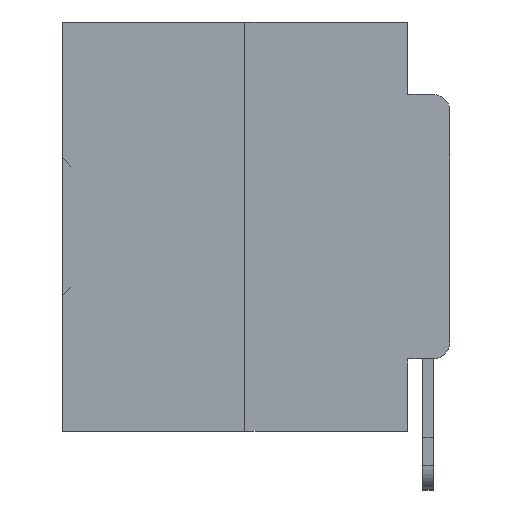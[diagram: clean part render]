
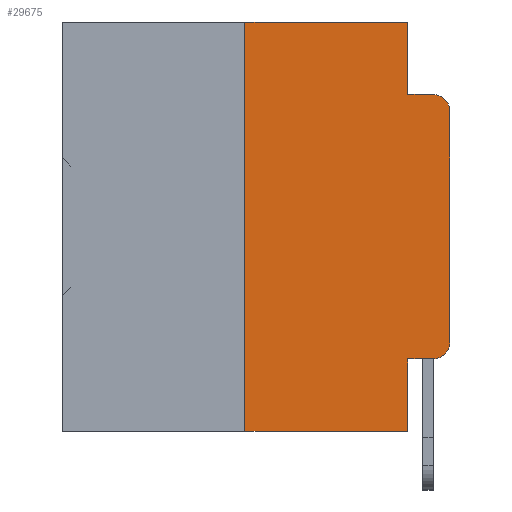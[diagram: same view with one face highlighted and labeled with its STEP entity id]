
A CAD part, left-side view. The second image highlights one B-rep face of the part: STEP entity #29675.
In plain terms, the highlighted planar face has unit normal (-1, 0, 0).
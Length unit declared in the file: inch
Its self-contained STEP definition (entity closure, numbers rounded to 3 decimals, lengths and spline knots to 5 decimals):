
#100 = DIRECTION ( 'NONE',  ( 0., 0., -1. ) ) ;
#539 = CIRCLE ( 'NONE', #15684, 0.02 ) ;
#1076 = CARTESIAN_POINT ( 'NONE',  ( 0., 0.051, 0. ) ) ;
#1246 = EDGE_CURVE ( 'NONE', #37813, #13424, #34353, .T. ) ;
#1493 = DIRECTION ( 'NONE',  ( 0., -1., 0. ) ) ;
#1650 = CARTESIAN_POINT ( 'NONE',  ( 0., 0.02, -0.0885 ) ) ;
#1823 = VERTEX_POINT ( 'NONE', #19265 ) ;
#1852 = ORIENTED_EDGE ( 'NONE', *, *, #6979, .F. ) ;
#2074 = CARTESIAN_POINT ( 'NONE',  ( 0., 0.25, -0.5 ) ) ;
#2303 = DIRECTION ( 'NONE',  ( 0., -1., 0. ) ) ;
#2508 = LINE ( 'NONE', #35994, #16537 ) ;
#2762 = ORIENTED_EDGE ( 'NONE', *, *, #8269, .T. ) ;
#3209 = DIRECTION ( 'NONE',  ( 0., 0., -1. ) ) ;
#4046 = DIRECTION ( 'NONE',  ( 0., 0., -1. ) ) ;
#4288 = ORIENTED_EDGE ( 'NONE', *, *, #35094, .T. ) ;
#4945 = EDGE_LOOP ( 'NONE', ( #7257, #2762, #1852, #21828, #7993, #10162, #32004, #15299, #10810, #4288 ) ) ;
#6101 = CARTESIAN_POINT ( 'NONE',  ( 0., 0.473, 0. ) ) ;
#6979 = EDGE_CURVE ( 'NONE', #8449, #25512, #19978, .T. ) ;
#7257 = ORIENTED_EDGE ( 'NONE', *, *, #22102, .T. ) ;
#7993 = ORIENTED_EDGE ( 'NONE', *, *, #1246, .F. ) ;
#8136 = LINE ( 'NONE', #26022, #16092 ) ;
#8179 = DIRECTION ( 'NONE',  ( 0., 0., 1. ) ) ;
#8269 = EDGE_CURVE ( 'NONE', #1823, #25512, #34664, .T. ) ;
#8449 = VERTEX_POINT ( 'NONE', #36029 ) ;
#10162 = ORIENTED_EDGE ( 'NONE', *, *, #11498, .F. ) ;
#10188 = CARTESIAN_POINT ( 'NONE',  ( 0., 0.473, -0.5 ) ) ;
#10362 = CARTESIAN_POINT ( 'NONE',  ( 0., 0.051, -0.4115 ) ) ;
#10559 = LINE ( 'NONE', #10188, #32386 ) ;
#10810 = ORIENTED_EDGE ( 'NONE', *, *, #13555, .T. ) ;
#11124 = VECTOR ( 'NONE', #14462, 39.37008 ) ;
#11498 = EDGE_CURVE ( 'NONE', #29410, #37813, #8136, .T. ) ;
#12300 = DIRECTION ( 'NONE',  ( 0., 0., 1. ) ) ;
#13424 = VERTEX_POINT ( 'NONE', #31315 ) ;
#13555 = EDGE_CURVE ( 'NONE', #15789, #35252, #35358, .T. ) ;
#14443 = CARTESIAN_POINT ( 'NONE',  ( 0., 0.02, -0.1085 ) ) ;
#14462 = DIRECTION ( 'NONE',  ( 0., -1., 0. ) ) ;
#15299 = ORIENTED_EDGE ( 'NONE', *, *, #35556, .F. ) ;
#15429 = VECTOR ( 'NONE', #100, 39.37008 ) ;
#15684 = AXIS2_PLACEMENT_3D ( 'NONE', #33490, #15753, #36446 ) ;
#15753 = DIRECTION ( 'NONE',  ( -1., 0., 0. ) ) ;
#15789 = VERTEX_POINT ( 'NONE', #10362 ) ;
#15991 = CARTESIAN_POINT ( 'NONE',  ( 0., 0.051, -0.0885 ) ) ;
#16077 = DIRECTION ( 'NONE',  ( 0., -1., 0. ) ) ;
#16092 = VECTOR ( 'NONE', #8179, 39.37008 ) ;
#16537 = VECTOR ( 'NONE', #12300, 39.37008 ) ;
#16777 = LINE ( 'NONE', #1076, #23718 ) ;
#17083 = AXIS2_PLACEMENT_3D ( 'NONE', #6101, #21064, #3209 ) ;
#17460 = DIRECTION ( 'NONE',  ( 0., 0., -1. ) ) ;
#18102 = PLANE ( 'NONE',  #17083 ) ;
#18538 = CARTESIAN_POINT ( 'NONE',  ( 0., 0.051, -0.5 ) ) ;
#19265 = CARTESIAN_POINT ( 'NONE',  ( 0., 0., -0.1085 ) ) ;
#19978 = LINE ( 'NONE', #15991, #11124 ) ;
#20208 = EDGE_CURVE ( 'NONE', #29410, #34433, #10559, .T. ) ;
#21064 = DIRECTION ( 'NONE',  ( 1., 0., 0. ) ) ;
#21828 = ORIENTED_EDGE ( 'NONE', *, *, #31117, .F. ) ;
#22102 = EDGE_CURVE ( 'NONE', #25591, #1823, #2508, .T. ) ;
#22750 = CARTESIAN_POINT ( 'NONE',  ( 0., 0., -0.3915 ) ) ;
#23718 = VECTOR ( 'NONE', #4046, 39.37008 ) ;
#25512 = VERTEX_POINT ( 'NONE', #1650 ) ;
#25591 = VERTEX_POINT ( 'NONE', #22750 ) ;
#25809 = CARTESIAN_POINT ( 'NONE',  ( 0., 0.25, 0. ) ) ;
#26022 = CARTESIAN_POINT ( 'NONE',  ( 0., 0.25, 0. ) ) ;
#26136 = CARTESIAN_POINT ( 'NONE',  ( 0., 0.051, -0.4115 ) ) ;
#26510 = VECTOR ( 'NONE', #1493, 39.37008 ) ;
#27007 = AXIS2_PLACEMENT_3D ( 'NONE', #14443, #35127, #17460 ) ;
#27542 = VECTOR ( 'NONE', #2303, 39.37008 ) ;
#29410 = VERTEX_POINT ( 'NONE', #2074 ) ;
#29675 = ADVANCED_FACE ( 'NONE', ( #36686 ), #18102, .F. ) ;
#30255 = LINE ( 'NONE', #35644, #15429 ) ;
#31117 = EDGE_CURVE ( 'NONE', #13424, #8449, #16777, .T. ) ;
#31315 = CARTESIAN_POINT ( 'NONE',  ( 0., 0.051, 0. ) ) ;
#32004 = ORIENTED_EDGE ( 'NONE', *, *, #20208, .T. ) ;
#32386 = VECTOR ( 'NONE', #16077, 39.37008 ) ;
#33490 = CARTESIAN_POINT ( 'NONE',  ( 0., 0.02, -0.3915 ) ) ;
#34353 = LINE ( 'NONE', #36062, #26510 ) ;
#34433 = VERTEX_POINT ( 'NONE', #18538 ) ;
#34664 = CIRCLE ( 'NONE', #27007, 0.02 ) ;
#35094 = EDGE_CURVE ( 'NONE', #35252, #25591, #539, .T. ) ;
#35127 = DIRECTION ( 'NONE',  ( -1., 0., 0. ) ) ;
#35252 = VERTEX_POINT ( 'NONE', #37079 ) ;
#35358 = LINE ( 'NONE', #26136, #27542 ) ;
#35556 = EDGE_CURVE ( 'NONE', #15789, #34433, #30255, .T. ) ;
#35644 = CARTESIAN_POINT ( 'NONE',  ( 0., 0.051, 0. ) ) ;
#35994 = CARTESIAN_POINT ( 'NONE',  ( 0., 0., 0. ) ) ;
#36029 = CARTESIAN_POINT ( 'NONE',  ( 0., 0.051, -0.0885 ) ) ;
#36062 = CARTESIAN_POINT ( 'NONE',  ( 0., 0.473, 0. ) ) ;
#36446 = DIRECTION ( 'NONE',  ( 0., 0., -1. ) ) ;
#36686 = FACE_OUTER_BOUND ( 'NONE', #4945, .T. ) ;
#37079 = CARTESIAN_POINT ( 'NONE',  ( 0., 0.02, -0.4115 ) ) ;
#37813 = VERTEX_POINT ( 'NONE', #25809 ) ;
